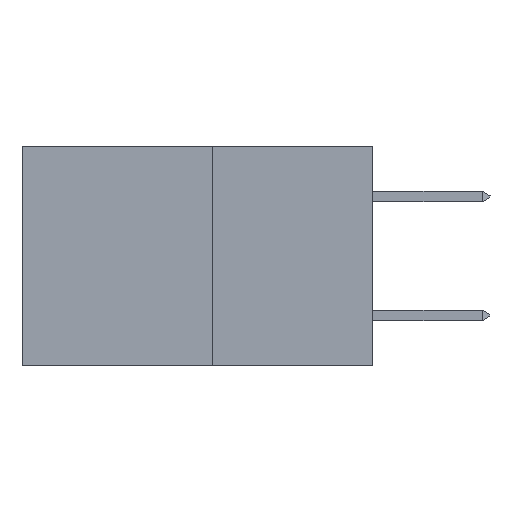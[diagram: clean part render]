
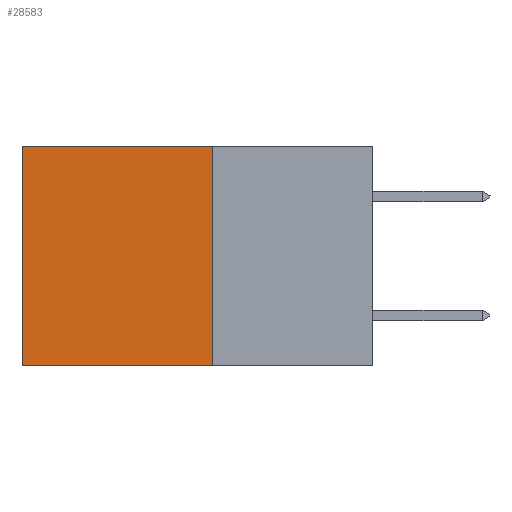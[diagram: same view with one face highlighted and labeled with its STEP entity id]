
A CAD part, left-side view. The second image highlights one B-rep face of the part: STEP entity #28583.
In plain terms, the highlighted planar face has unit normal (-1, 0, 0).
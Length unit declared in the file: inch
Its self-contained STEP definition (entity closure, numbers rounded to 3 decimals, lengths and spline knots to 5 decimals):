
#717 = DIRECTION ( 'NONE',  ( 0., 0., -1. ) ) ;
#4999 = CARTESIAN_POINT ( 'NONE',  ( 0.277, 0.59, -0.37 ) ) ;
#5086 = ORIENTED_EDGE ( 'NONE', *, *, #16661, .F. ) ;
#5407 = VERTEX_POINT ( 'NONE', #15506 ) ;
#7027 = VERTEX_POINT ( 'NONE', #4999 ) ;
#8318 = DIRECTION ( 'NONE',  ( 0., 1., 0. ) ) ;
#9127 = CARTESIAN_POINT ( 'NONE',  ( 0.277, 0.27, 0. ) ) ;
#9796 = LINE ( 'NONE', #18137, #23367 ) ;
#10936 = ORIENTED_EDGE ( 'NONE', *, *, #32924, .T. ) ;
#11081 = VERTEX_POINT ( 'NONE', #9127 ) ;
#12067 = DIRECTION ( 'NONE',  ( 1., 0., 0. ) ) ;
#12711 = VECTOR ( 'NONE', #8318, 39.37008 ) ;
#15469 = VERTEX_POINT ( 'NONE', #32246 ) ;
#15506 = CARTESIAN_POINT ( 'NONE',  ( 0.277, 0.27, -0.37 ) ) ;
#15856 = ORIENTED_EDGE ( 'NONE', *, *, #23257, .F. ) ;
#16661 = EDGE_CURVE ( 'NONE', #11081, #5407, #33288, .T. ) ;
#18137 = CARTESIAN_POINT ( 'NONE',  ( 0.277, 0.27, 0. ) ) ;
#18324 = ORIENTED_EDGE ( 'NONE', *, *, #30647, .T. ) ;
#19037 = LINE ( 'NONE', #24540, #12711 ) ;
#20100 = CARTESIAN_POINT ( 'NONE',  ( 0.277, 0.27, -0.37 ) ) ;
#20910 = DIRECTION ( 'NONE',  ( 0., 1., 0. ) ) ;
#23257 = EDGE_CURVE ( 'NONE', #5407, #7027, #19037, .T. ) ;
#23367 = VECTOR ( 'NONE', #20910, 39.37008 ) ;
#23438 = FACE_OUTER_BOUND ( 'NONE', #27399, .T. ) ;
#24540 = CARTESIAN_POINT ( 'NONE',  ( 0.277, 0.27, -0.37 ) ) ;
#25439 = VECTOR ( 'NONE', #31548, 39.37008 ) ;
#27399 = EDGE_LOOP ( 'NONE', ( #18324, #15856, #5086, #10936 ) ) ;
#28181 = PLANE ( 'NONE',  #32789 ) ;
#28583 = ADVANCED_FACE ( 'NONE', ( #23438 ), #28181, .F. ) ;
#28898 = CARTESIAN_POINT ( 'NONE',  ( 0.277, 0.27, -0.37 ) ) ;
#30647 = EDGE_CURVE ( 'NONE', #15469, #7027, #32139, .T. ) ;
#30845 = DIRECTION ( 'NONE',  ( 0., 0., -1. ) ) ;
#31307 = VECTOR ( 'NONE', #717, 39.37008 ) ;
#31548 = DIRECTION ( 'NONE',  ( 0., 0., -1. ) ) ;
#32139 = LINE ( 'NONE', #33043, #31307 ) ;
#32246 = CARTESIAN_POINT ( 'NONE',  ( 0.277, 0.59, 0. ) ) ;
#32789 = AXIS2_PLACEMENT_3D ( 'NONE', #20100, #12067, #30845 ) ;
#32924 = EDGE_CURVE ( 'NONE', #11081, #15469, #9796, .T. ) ;
#33043 = CARTESIAN_POINT ( 'NONE',  ( 0.277, 0.59, -0.37 ) ) ;
#33288 = LINE ( 'NONE', #28898, #25439 ) ;
